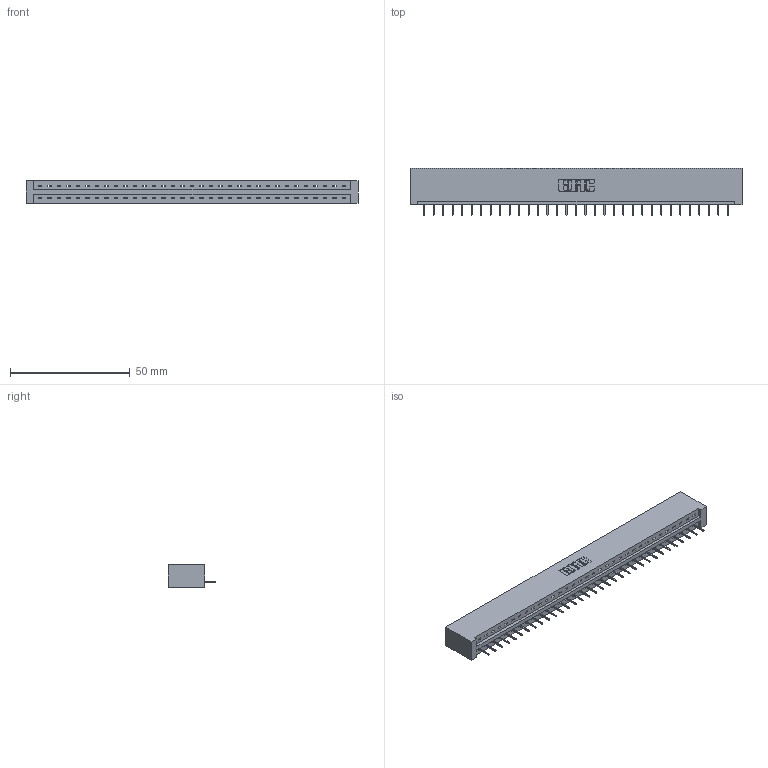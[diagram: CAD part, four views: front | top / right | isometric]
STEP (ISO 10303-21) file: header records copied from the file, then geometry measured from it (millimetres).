
FILE_DESCRIPTION (( 'STEP AP203' ), '1' );
FILE_NAME ('387-033-524-101.STEP', '2019-10-03T21:50:54', ( '' ), ( '' ), 'SwSTEP 2.0', 'SolidWorks 2016', '' );
FILE_SCHEMA (( 'CONFIG_CONTROL_DESIGN' ));
Length unit declared in the file: inch
Products named in the file (3): 337 Part_No Mounting Lugs; 387-033-524-101; 345-292-001_345-293-124
Assembly tree (34 placements, depth 2):
  387-033-524-101
    337 Part_No Mounting Lugs
    345-292-001_345-293-124  x33
Bounding box: 138.63 x 19.69 x 9.4 mm (x, y, z)
Volume: 14904.3 mm3; surface area: 14874.5 mm2
Topology: 34 solids, 34 shells, 2284 faces, 6623 edges, 4282 vertices
Faces by surface type: plane 1782, cylinder 502
Entity records: 25491 total; most frequent: CARTESIAN_POINT 4445, ORIENTED_EDGE 4414, DIRECTION 3753, EDGE_CURVE 2207, VECTOR 2091, LINE 2091, VERTEX_POINT 1466, AXIS2_PLACEMENT_3D 831
